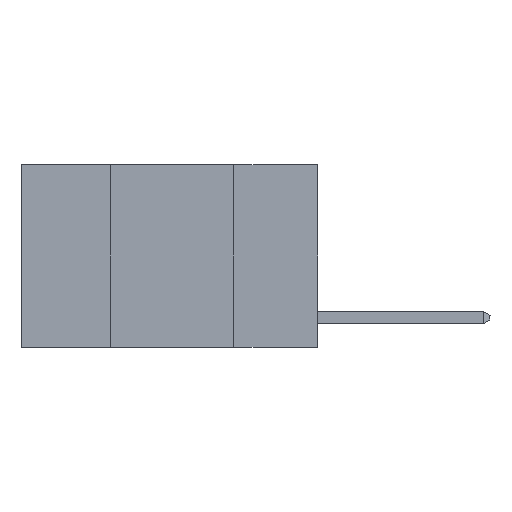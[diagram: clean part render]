
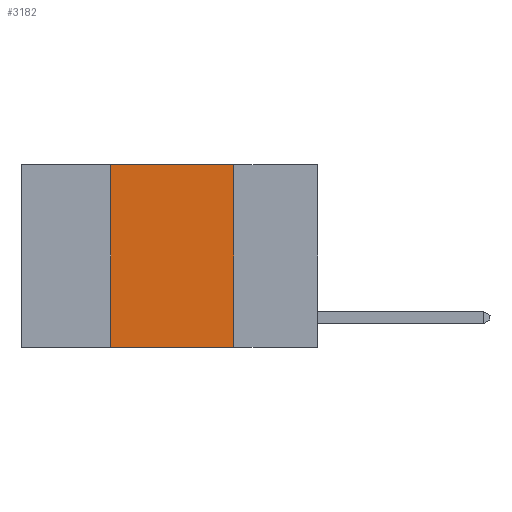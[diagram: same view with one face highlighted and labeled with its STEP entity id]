
A CAD part, left-side view. The second image highlights one B-rep face of the part: STEP entity #3182.
In plain terms, the highlighted planar face has unit normal (-1, 0, 0).
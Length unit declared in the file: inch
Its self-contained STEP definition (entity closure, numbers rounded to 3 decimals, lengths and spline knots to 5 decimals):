
#383 = LINE ( 'NONE', #13340, #11324 ) ;
#971 = VECTOR ( 'NONE', #4802, 39.37008 ) ;
#1241 = DIRECTION ( 'NONE',  ( 0., -1., 0. ) ) ;
#2858 = VECTOR ( 'NONE', #9664, 39.37008 ) ;
#3082 = EDGE_CURVE ( 'NONE', #18347, #20455, #25479, .T. ) ;
#3182 = ADVANCED_FACE ( 'NONE', ( #5895 ), #16463, .F. ) ;
#3363 = CARTESIAN_POINT ( 'NONE',  ( 0., 0.42, 0. ) ) ;
#4802 = DIRECTION ( 'NONE',  ( 0., 0., -1. ) ) ;
#5599 = CARTESIAN_POINT ( 'NONE',  ( 0., 0.6, 0. ) ) ;
#5895 = FACE_OUTER_BOUND ( 'NONE', #27455, .T. ) ;
#7705 = VERTEX_POINT ( 'NONE', #13343 ) ;
#9664 = DIRECTION ( 'NONE',  ( 0., 0., 1. ) ) ;
#9945 = DIRECTION ( 'NONE',  ( 1., 0., 0. ) ) ;
#11324 = VECTOR ( 'NONE', #15528, 39.37008 ) ;
#11913 = LINE ( 'NONE', #20016, #971 ) ;
#12241 = AXIS2_PLACEMENT_3D ( 'NONE', #20860, #9945, #25306 ) ;
#12266 = VECTOR ( 'NONE', #1241, 39.37008 ) ;
#13340 = CARTESIAN_POINT ( 'NONE',  ( 0., 0.6, -0.37 ) ) ;
#13343 = CARTESIAN_POINT ( 'NONE',  ( 0., 0.17, 0. ) ) ;
#13394 = ORIENTED_EDGE ( 'NONE', *, *, #18089, .F. ) ;
#15528 = DIRECTION ( 'NONE',  ( 0., -1., 0. ) ) ;
#16463 = PLANE ( 'NONE',  #12241 ) ;
#17316 = CARTESIAN_POINT ( 'NONE',  ( 0., 0.42, -0.37 ) ) ;
#17857 = ORIENTED_EDGE ( 'NONE', *, *, #23111, .F. ) ;
#18089 = EDGE_CURVE ( 'NONE', #20455, #7705, #23262, .T. ) ;
#18347 = VERTEX_POINT ( 'NONE', #17316 ) ;
#19186 = ORIENTED_EDGE ( 'NONE', *, *, #3082, .F. ) ;
#19794 = CARTESIAN_POINT ( 'NONE',  ( 0., 0.17, -0.37 ) ) ;
#20016 = CARTESIAN_POINT ( 'NONE',  ( 0., 0.17, 0. ) ) ;
#20455 = VERTEX_POINT ( 'NONE', #3363 ) ;
#20843 = EDGE_CURVE ( 'NONE', #18347, #25535, #383, .T. ) ;
#20860 = CARTESIAN_POINT ( 'NONE',  ( 0., 0.6, 0. ) ) ;
#22824 = CARTESIAN_POINT ( 'NONE',  ( 0., 0.42, 0. ) ) ;
#23111 = EDGE_CURVE ( 'NONE', #7705, #25535, #11913, .T. ) ;
#23262 = LINE ( 'NONE', #5599, #12266 ) ;
#25063 = ORIENTED_EDGE ( 'NONE', *, *, #20843, .T. ) ;
#25306 = DIRECTION ( 'NONE',  ( 0., 0., -1. ) ) ;
#25479 = LINE ( 'NONE', #22824, #2858 ) ;
#25535 = VERTEX_POINT ( 'NONE', #19794 ) ;
#27455 = EDGE_LOOP ( 'NONE', ( #17857, #13394, #19186, #25063 ) ) ;
